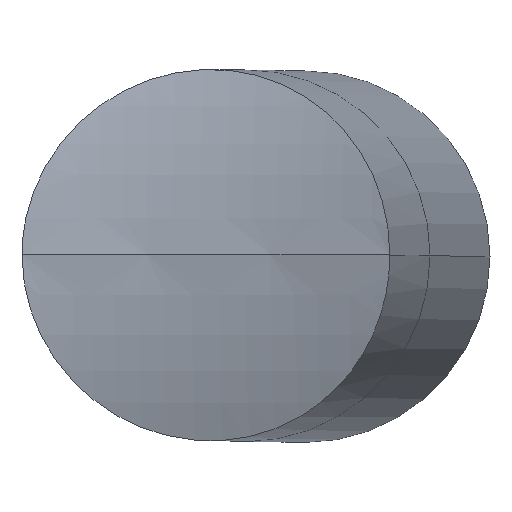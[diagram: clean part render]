
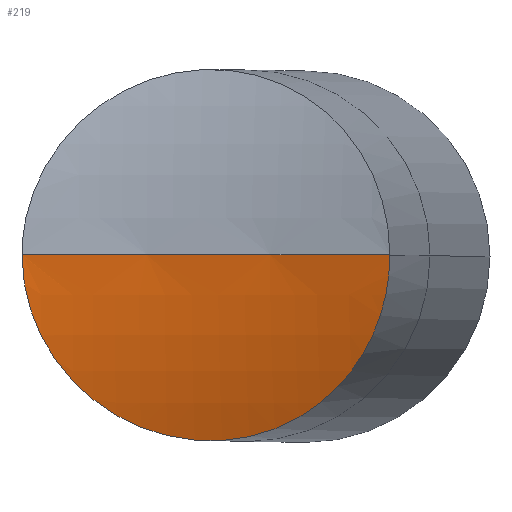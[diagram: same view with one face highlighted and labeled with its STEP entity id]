
A CAD part, top view. The second image highlights one B-rep face of the part: STEP entity #219.
In plain terms, the highlighted toroidal (fillet/blend) face has major radius 28.088 mm and minor radius 11.5 mm.
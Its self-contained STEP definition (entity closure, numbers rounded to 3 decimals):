
#2 = VERTEX_POINT ( 'NONE', #41 ) ;
#4 = B_SPLINE_CURVE_WITH_KNOTS ( 'NONE', 3,
 ( #97, #233, #270, #102, #114 ),
 .UNSPECIFIED., .F., .F.,
 ( 4, 1, 4 ),
 ( 0.012, 0.012, 0.012 ),
 .UNSPECIFIED. ) ;
#7 = EDGE_CURVE ( 'NONE', #2, #169, #68, .T. ) ;
#11 = CARTESIAN_POINT ( 'NONE',  ( -11.965, 15.494, 15.822 ) ) ;
#15 = AXIS2_PLACEMENT_3D ( 'NONE', #76, #67, #80 ) ;
#18 = CARTESIAN_POINT ( 'NONE',  ( -5.55, 15.495, 16.749 ) ) ;
#29 = EDGE_CURVE ( 'NONE', #190, #158, #4, .T. ) ;
#41 = CARTESIAN_POINT ( 'NONE',  ( -5.55, 15.494, 16.749 ) ) ;
#42 = CARTESIAN_POINT ( 'NONE',  ( -11.086, 15.503, 32.386 ) ) ;
#44 = DIRECTION ( 'NONE',  ( 0., 1., 0. ) ) ;
#50 = B_SPLINE_CURVE_WITH_KNOTS ( 'NONE', 3,
 ( #11, #284, #280, #278, #276, #275, #272, #267, #263, #262, #261, #260, #259, #257, #256, #250, #247, #245, #242, #241, #239, #229, #223, #202, #201, #193, #186, #183, #171, #163, #150, #149 ),
 .UNSPECIFIED., .F., .F.,
 ( 4, 2, 2, 2, 2, 2, 2, 2, 2, 2, 2, 2, 2, 2, 2, 4 ),
 ( 0.012, 0.013, 0.014, 0.014, 0.015, 0.016, 0.016, 0.017, 0.018, 0.018, 0.019, 0.02, 0.021, 0.021, 0.022, 0.023 ),
 .UNSPECIFIED. ) ;
#53 = DIRECTION ( 'NONE',  ( 1., 0., 0. ) ) ;
#55 = AXIS2_PLACEMENT_3D ( 'NONE', #42, #44, #53 ) ;
#62 = ORIENTED_EDGE ( 'NONE', *, *, #283, .T. ) ;
#67 = DIRECTION ( 'NONE',  ( 0., 1., 0. ) ) ;
#68 = B_SPLINE_CURVE_WITH_KNOTS ( 'NONE', 3,
 ( #81, #18, #164, #132, #156 ),
 .UNSPECIFIED., .F., .F.,
 ( 4, 1, 4 ),
 ( 0.002, 0.002, 0.002 ),
 .UNSPECIFIED. ) ;
#73 = CARTESIAN_POINT ( 'NONE',  ( -11.965, 15.503, 15.822 ) ) ;
#76 = CARTESIAN_POINT ( 'NONE',  ( -11.086, 15.503, 32.386 ) ) ;
#80 = DIRECTION ( 'NONE',  ( 0., 0., 1. ) ) ;
#81 = CARTESIAN_POINT ( 'NONE',  ( -5.55, 15.494, 16.749 ) ) ;
#97 = CARTESIAN_POINT ( 'NONE',  ( -11.965, 15.503, 15.822 ) ) ;
#102 = CARTESIAN_POINT ( 'NONE',  ( -11.965, 15.495, 15.822 ) ) ;
#114 = CARTESIAN_POINT ( 'NONE',  ( -11.965, 15.494, 15.822 ) ) ;
#132 = CARTESIAN_POINT ( 'NONE',  ( -5.55, 15.502, 16.749 ) ) ;
#134 = TOROIDAL_SURFACE ( 'NONE', #55, 28.088, 11.5 ) ;
#137 = CIRCLE ( 'NONE', #15, 16.588 ) ;
#139 = ORIENTED_EDGE ( 'NONE', *, *, #7, .T. ) ;
#149 = CARTESIAN_POINT ( 'NONE',  ( -5.55, 15.494, 16.749 ) ) ;
#150 = CARTESIAN_POINT ( 'NONE',  ( -5.55, 15.278, 16.749 ) ) ;
#156 = CARTESIAN_POINT ( 'NONE',  ( -5.55, 15.503, 16.749 ) ) ;
#158 = VERTEX_POINT ( 'NONE', #214 ) ;
#162 = EDGE_CURVE ( 'NONE', #169, #190, #137, .T. ) ;
#163 = CARTESIAN_POINT ( 'NONE',  ( -5.571, 15.063, 16.735 ) ) ;
#164 = CARTESIAN_POINT ( 'NONE',  ( -5.55, 15.498, 16.749 ) ) ;
#169 = VERTEX_POINT ( 'NONE', #269 ) ;
#171 = CARTESIAN_POINT ( 'NONE',  ( -5.649, 14.647, 16.683 ) ) ;
#173 = ORIENTED_EDGE ( 'NONE', *, *, #162, .T. ) ;
#182 = ORIENTED_EDGE ( 'NONE', *, *, #29, .T. ) ;
#183 = CARTESIAN_POINT ( 'NONE',  ( -5.709, 14.441, 16.644 ) ) ;
#186 = CARTESIAN_POINT ( 'NONE',  ( -5.862, 14.05, 16.547 ) ) ;
#190 = VERTEX_POINT ( 'NONE', #73 ) ;
#193 = CARTESIAN_POINT ( 'NONE',  ( -5.956, 13.867, 16.49 ) ) ;
#201 = CARTESIAN_POINT ( 'NONE',  ( -6.175, 13.52, 16.363 ) ) ;
#202 = CARTESIAN_POINT ( 'NONE',  ( -6.302, 13.357, 16.293 ) ) ;
#204 = EDGE_LOOP ( 'NONE', ( #139, #173, #182, #62 ) ) ;
#214 = CARTESIAN_POINT ( 'NONE',  ( -11.965, 15.494, 15.822 ) ) ;
#219 = ADVANCED_FACE ( 'NONE', ( #258 ), #134, .T. ) ;
#223 = CARTESIAN_POINT ( 'NONE',  ( -6.724, 12.913, 16.077 ) ) ;
#229 = CARTESIAN_POINT ( 'NONE',  ( -7.059, 12.676, 15.928 ) ) ;
#233 = CARTESIAN_POINT ( 'NONE',  ( -11.965, 15.502, 15.822 ) ) ;
#239 = CARTESIAN_POINT ( 'NONE',  ( -7.626, 12.429, 15.735 ) ) ;
#241 = CARTESIAN_POINT ( 'NONE',  ( -7.823, 12.366, 15.677 ) ) ;
#242 = CARTESIAN_POINT ( 'NONE',  ( -8.232, 12.279, 15.577 ) ) ;
#245 = CARTESIAN_POINT ( 'NONE',  ( -8.446, 12.257, 15.535 ) ) ;
#247 = CARTESIAN_POINT ( 'NONE',  ( -8.869, 12.254, 15.473 ) ) ;
#250 = CARTESIAN_POINT ( 'NONE',  ( -9.082, 12.274, 15.453 ) ) ;
#256 = CARTESIAN_POINT ( 'NONE',  ( -9.508, 12.357, 15.432 ) ) ;
#257 = CARTESIAN_POINT ( 'NONE',  ( -9.713, 12.419, 15.432 ) ) ;
#258 = FACE_OUTER_BOUND ( 'NONE', #204, .T. ) ;
#259 = CARTESIAN_POINT ( 'NONE',  ( -10.108, 12.581, 15.448 ) ) ;
#260 = CARTESIAN_POINT ( 'NONE',  ( -10.3, 12.682, 15.465 ) ) ;
#261 = CARTESIAN_POINT ( 'NONE',  ( -10.659, 12.916, 15.509 ) ) ;
#262 = CARTESIAN_POINT ( 'NONE',  ( -10.825, 13.049, 15.536 ) ) ;
#263 = CARTESIAN_POINT ( 'NONE',  ( -11.13, 13.345, 15.594 ) ) ;
#267 = CARTESIAN_POINT ( 'NONE',  ( -11.271, 13.509, 15.626 ) ) ;
#269 = CARTESIAN_POINT ( 'NONE',  ( -5.55, 15.503, 16.749 ) ) ;
#270 = CARTESIAN_POINT ( 'NONE',  ( -11.965, 15.498, 15.822 ) ) ;
#272 = CARTESIAN_POINT ( 'NONE',  ( -11.513, 13.858, 15.687 ) ) ;
#275 = CARTESIAN_POINT ( 'NONE',  ( -11.618, 14.044, 15.715 ) ) ;
#276 = CARTESIAN_POINT ( 'NONE',  ( -11.789, 14.439, 15.765 ) ) ;
#278 = CARTESIAN_POINT ( 'NONE',  ( -11.855, 14.643, 15.786 ) ) ;
#280 = CARTESIAN_POINT ( 'NONE',  ( -11.943, 15.061, 15.814 ) ) ;
#283 = EDGE_CURVE ( 'NONE', #158, #2, #50, .T. ) ;
#284 = CARTESIAN_POINT ( 'NONE',  ( -11.965, 15.279, 15.822 ) ) ;
